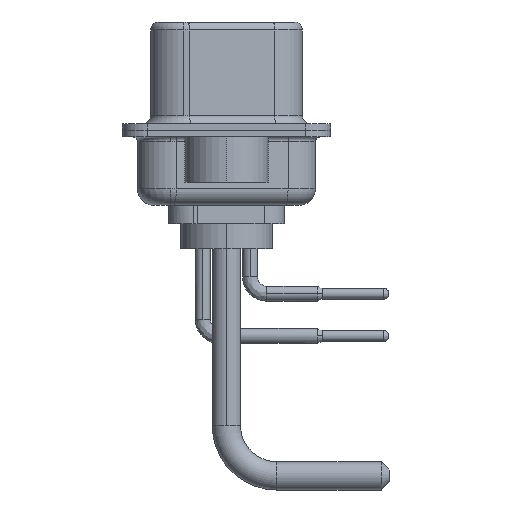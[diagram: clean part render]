
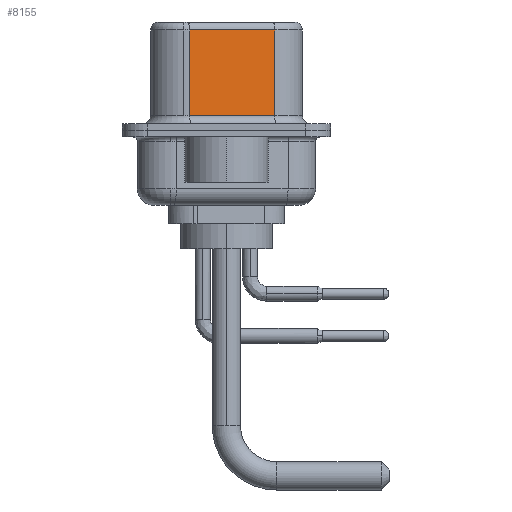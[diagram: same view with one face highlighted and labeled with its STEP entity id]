
A CAD part, left-side view. The second image highlights one B-rep face of the part: STEP entity #8155.
In plain terms, the highlighted planar face has unit normal (-0.985, -0.174, 0).
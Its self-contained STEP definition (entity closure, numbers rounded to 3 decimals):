
#26 = CARTESIAN_POINT ( 'NONE',  ( 4.58, -2.897, 6.02 ) ) ;
#688 = DIRECTION ( 'NONE',  ( 0.174, -0.985, 0. ) ) ;
#1346 = EDGE_CURVE ( 'NONE', #4012, #14126, #18213, .T. ) ;
#1933 = CARTESIAN_POINT ( 'NONE',  ( 3.68, 2.203, 6.02 ) ) ;
#3504 = ORIENTED_EDGE ( 'NONE', *, *, #9144, .T. ) ;
#3946 = ORIENTED_EDGE ( 'NONE', *, *, #19397, .T. ) ;
#4012 = VERTEX_POINT ( 'NONE', #9023 ) ;
#5054 = DIRECTION ( 'NONE',  ( 0., 0., -1. ) ) ;
#5219 = DIRECTION ( 'NONE',  ( 0., 0., -1. ) ) ;
#5353 = LINE ( 'NONE', #14148, #6977 ) ;
#5614 = AXIS2_PLACEMENT_3D ( 'NONE', #26492, #9030, #13352 ) ;
#6713 = FACE_OUTER_BOUND ( 'NONE', #22793, .T. ) ;
#6977 = VECTOR ( 'NONE', #5219, 1000. ) ;
#8155 = ADVANCED_FACE ( 'NONE', ( #6713 ), #17728, .F. ) ;
#9023 = CARTESIAN_POINT ( 'NONE',  ( 3.68, 2.203, 0.9 ) ) ;
#9030 = DIRECTION ( 'NONE',  ( 0.985, 0.174, 0. ) ) ;
#9105 = LINE ( 'NONE', #27284, #11678 ) ;
#9144 = EDGE_CURVE ( 'NONE', #27789, #25479, #12764, .T. ) ;
#11110 = CARTESIAN_POINT ( 'NONE',  ( 4.58, -2.897, 0.9 ) ) ;
#11203 = EDGE_CURVE ( 'NONE', #27789, #14126, #5353, .T. ) ;
#11656 = VECTOR ( 'NONE', #23620, 1000. ) ;
#11678 = VECTOR ( 'NONE', #5054, 1000. ) ;
#12764 = LINE ( 'NONE', #26, #11656 ) ;
#12789 = CARTESIAN_POINT ( 'NONE',  ( 4.58, -2.897, 6.02 ) ) ;
#13352 = DIRECTION ( 'NONE',  ( -0.174, 0.985, 0. ) ) ;
#14126 = VERTEX_POINT ( 'NONE', #14622 ) ;
#14148 = CARTESIAN_POINT ( 'NONE',  ( 4.58, -2.897, 6.52 ) ) ;
#14622 = CARTESIAN_POINT ( 'NONE',  ( 4.58, -2.897, 0.9 ) ) ;
#14966 = VECTOR ( 'NONE', #688, 1000. ) ;
#15757 = ORIENTED_EDGE ( 'NONE', *, *, #11203, .F. ) ;
#17329 = ORIENTED_EDGE ( 'NONE', *, *, #1346, .T. ) ;
#17728 = PLANE ( 'NONE',  #5614 ) ;
#18213 = LINE ( 'NONE', #11110, #14966 ) ;
#19397 = EDGE_CURVE ( 'NONE', #25479, #4012, #9105, .T. ) ;
#22793 = EDGE_LOOP ( 'NONE', ( #15757, #3504, #3946, #17329 ) ) ;
#23620 = DIRECTION ( 'NONE',  ( -0.174, 0.985, 0. ) ) ;
#25479 = VERTEX_POINT ( 'NONE', #1933 ) ;
#26492 = CARTESIAN_POINT ( 'NONE',  ( 4.58, -2.897, 6.52 ) ) ;
#27284 = CARTESIAN_POINT ( 'NONE',  ( 3.68, 2.203, 6.52 ) ) ;
#27789 = VERTEX_POINT ( 'NONE', #12789 ) ;
